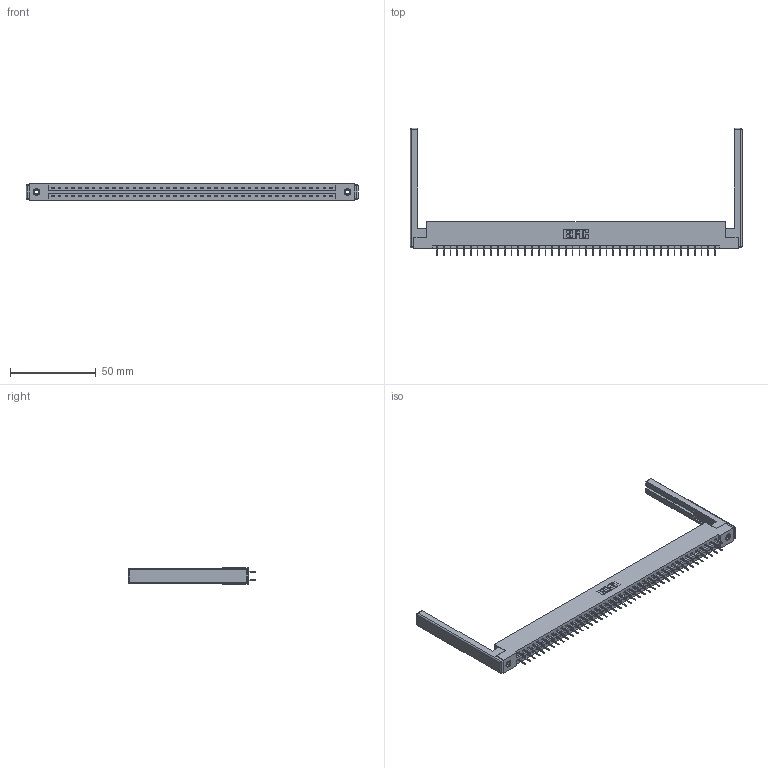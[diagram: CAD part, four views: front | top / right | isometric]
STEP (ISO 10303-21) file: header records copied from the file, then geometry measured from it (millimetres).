
FILE_DESCRIPTION (( 'STEP AP203' ), '1' );
FILE_NAME ('387-084-524-268.STEP', '2019-10-23T01:13:54', ( '' ), ( '' ), 'SwSTEP 2.0', 'SolidWorks 2016', '' );
FILE_SCHEMA (( 'CONFIG_CONTROL_DESIGN' ));
Length unit declared in the file: inch
Products named in the file (5): 337 Part_Flush Mounting Lugs - 0.156 Dia-TI; 345-292-001_345-293-124; 387-084-524-268; 345-250-001_345-250-001-102; 307-220-068
Assembly tree (89 placements, depth 2):
  387-084-524-268
    337 Part_Flush Mounting Lugs - 0.156 Dia-TI
    345-292-001_345-293-124  x84
    345-250-001_345-250-001-102  x2
    307-220-068  x2
Bounding box: 193.85 x 74.43 x 9.4 mm (x, y, z)
Volume: 24687.4 mm3; surface area: 26592.8 mm2
Topology: 89 solids, 89 shells, 5140 faces, 14561 edges, 9350 vertices
Faces by surface type: plane 3854, cylinder 1262, cone 12, sphere 8, torus 4
Entity records: 35398 total; most frequent: CARTESIAN_POINT 5927, ORIENTED_EDGE 5852, DIRECTION 5112, EDGE_CURVE 2926, LINE 2752, VECTOR 2752, VERTEX_POINT 1938, AXIS2_PLACEMENT_3D 1180
